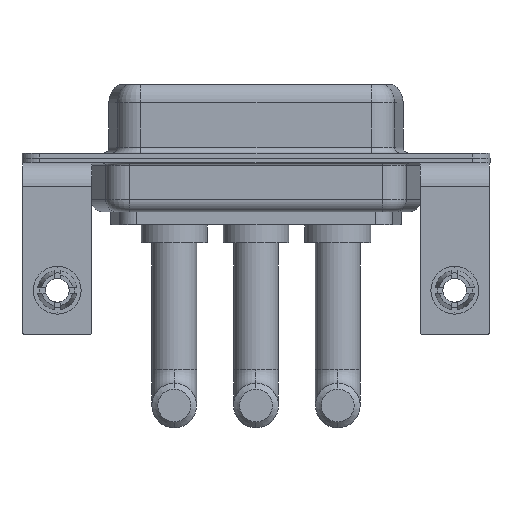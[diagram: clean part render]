
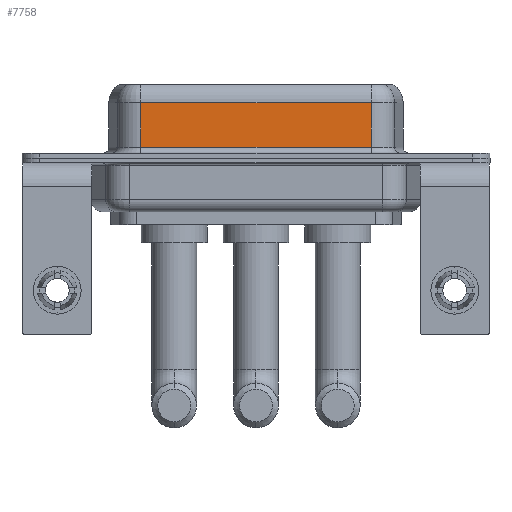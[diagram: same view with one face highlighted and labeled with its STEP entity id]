
A CAD part, front view. The second image highlights one B-rep face of the part: STEP entity #7758.
In plain terms, the highlighted planar face has unit normal (0, -1, 0).
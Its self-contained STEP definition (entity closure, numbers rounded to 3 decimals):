
#1056 = CARTESIAN_POINT ( 'NONE',  ( 26.287, -3.95, 6.4 ) ) ;
#2414 = CARTESIAN_POINT ( 'NONE',  ( 26.287, -3.95, 4.65 ) ) ;
#3083 = PLANE ( 'NONE',  #8774 ) ;
#3388 = DIRECTION ( 'NONE',  ( -1., 0., 0. ) ) ;
#3703 = LINE ( 'NONE', #13844, #14194 ) ;
#3768 = VERTEX_POINT ( 'NONE', #5782 ) ;
#3839 = ORIENTED_EDGE ( 'NONE', *, *, #14214, .T. ) ;
#4261 = DIRECTION ( 'NONE',  ( 0., 0., 1. ) ) ;
#4340 = EDGE_CURVE ( 'NONE', #11433, #4978, #11456, .T. ) ;
#4898 = CARTESIAN_POINT ( 'NONE',  ( 26.287, -3.95, 0.9 ) ) ;
#4978 = VERTEX_POINT ( 'NONE', #8714 ) ;
#5726 = EDGE_CURVE ( 'NONE', #4978, #3768, #3703, .T. ) ;
#5782 = CARTESIAN_POINT ( 'NONE',  ( 7.013, -3.95, 0.9 ) ) ;
#6195 = LINE ( 'NONE', #7527, #13066 ) ;
#7461 = ORIENTED_EDGE ( 'NONE', *, *, #5726, .T. ) ;
#7527 = CARTESIAN_POINT ( 'NONE',  ( 26.287, -3.95, 0.9 ) ) ;
#7691 = DIRECTION ( 'NONE',  ( 0., 1., 0. ) ) ;
#7758 = ADVANCED_FACE ( 'NONE', ( #8744 ), #3083, .F. ) ;
#7932 = CARTESIAN_POINT ( 'NONE',  ( 26.287, -3.95, 6.4 ) ) ;
#8080 = DIRECTION ( 'NONE',  ( 0., 0., -1. ) ) ;
#8513 = VECTOR ( 'NONE', #8080, 1000. ) ;
#8536 = ORIENTED_EDGE ( 'NONE', *, *, #9460, .F. ) ;
#8714 = CARTESIAN_POINT ( 'NONE',  ( 7.013, -3.95, 4.65 ) ) ;
#8744 = FACE_OUTER_BOUND ( 'NONE', #12252, .T. ) ;
#8774 = AXIS2_PLACEMENT_3D ( 'NONE', #1056, #7691, #4261 ) ;
#8976 = LINE ( 'NONE', #7932, #8513 ) ;
#9460 = EDGE_CURVE ( 'NONE', #11433, #12326, #8976, .T. ) ;
#9703 = DIRECTION ( 'NONE',  ( 1., 0., 0. ) ) ;
#10674 = CARTESIAN_POINT ( 'NONE',  ( 26.287, -3.95, 4.65 ) ) ;
#11433 = VERTEX_POINT ( 'NONE', #10674 ) ;
#11456 = LINE ( 'NONE', #2414, #13204 ) ;
#12252 = EDGE_LOOP ( 'NONE', ( #8536, #14482, #7461, #3839 ) ) ;
#12326 = VERTEX_POINT ( 'NONE', #4898 ) ;
#12880 = DIRECTION ( 'NONE',  ( 0., 0., -1. ) ) ;
#13066 = VECTOR ( 'NONE', #9703, 1000. ) ;
#13204 = VECTOR ( 'NONE', #3388, 1000. ) ;
#13844 = CARTESIAN_POINT ( 'NONE',  ( 7.013, -3.95, 6.4 ) ) ;
#14194 = VECTOR ( 'NONE', #12880, 1000. ) ;
#14214 = EDGE_CURVE ( 'NONE', #3768, #12326, #6195, .T. ) ;
#14482 = ORIENTED_EDGE ( 'NONE', *, *, #4340, .T. ) ;
